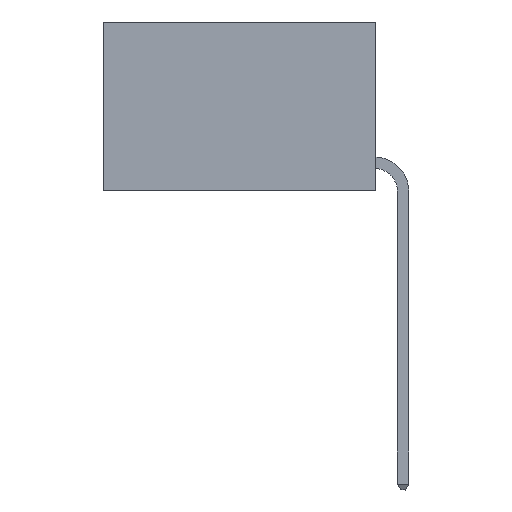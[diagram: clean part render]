
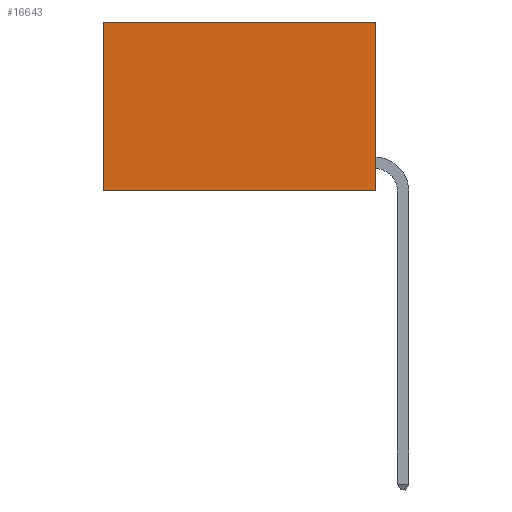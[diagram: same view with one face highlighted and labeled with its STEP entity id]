
A CAD part, left-side view. The second image highlights one B-rep face of the part: STEP entity #16643.
In plain terms, the highlighted planar face has unit normal (-1, 0, 0).
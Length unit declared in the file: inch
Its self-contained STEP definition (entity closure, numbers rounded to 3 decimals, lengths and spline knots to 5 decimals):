
#295 = DIRECTION ( 'NONE',  ( 0., 0., -1. ) ) ;
#575 = VECTOR ( 'NONE', #19983, 39.37008 ) ;
#741 = CARTESIAN_POINT ( 'NONE',  ( 0.2625, 0.6, 0. ) ) ;
#855 = VERTEX_POINT ( 'NONE', #15680 ) ;
#1957 = CARTESIAN_POINT ( 'NONE',  ( 0.2625, 0., 0. ) ) ;
#2111 = EDGE_CURVE ( 'NONE', #17604, #12162, #2617, .T. ) ;
#2617 = LINE ( 'NONE', #741, #11077 ) ;
#3905 = VECTOR ( 'NONE', #17880, 39.37008 ) ;
#4151 = EDGE_CURVE ( 'NONE', #9813, #855, #12773, .T. ) ;
#4707 = CARTESIAN_POINT ( 'NONE',  ( 0.2625, 0., 0. ) ) ;
#5472 = PLANE ( 'NONE',  #5773 ) ;
#5773 = AXIS2_PLACEMENT_3D ( 'NONE', #20198, #10527, #295 ) ;
#5957 = VECTOR ( 'NONE', #14330, 39.37008 ) ;
#5994 = DIRECTION ( 'NONE',  ( 0., 0., -1. ) ) ;
#7853 = CARTESIAN_POINT ( 'NONE',  ( 0.2625, 0.6, -0.37 ) ) ;
#7893 = CARTESIAN_POINT ( 'NONE',  ( 0.2625, 0.6, 0. ) ) ;
#8327 = EDGE_LOOP ( 'NONE', ( #21226, #11391, #18848, #16035 ) ) ;
#8675 = CARTESIAN_POINT ( 'NONE',  ( 0.2625, 0., -0.37 ) ) ;
#9660 = FACE_OUTER_BOUND ( 'NONE', #8327, .T. ) ;
#9813 = VERTEX_POINT ( 'NONE', #1957 ) ;
#10527 = DIRECTION ( 'NONE',  ( 1., 0., 0. ) ) ;
#11077 = VECTOR ( 'NONE', #5994, 39.37008 ) ;
#11391 = ORIENTED_EDGE ( 'NONE', *, *, #15274, .F. ) ;
#12162 = VERTEX_POINT ( 'NONE', #7853 ) ;
#12773 = LINE ( 'NONE', #4707, #3905 ) ;
#14330 = DIRECTION ( 'NONE',  ( 0., 1., 0. ) ) ;
#15274 = EDGE_CURVE ( 'NONE', #855, #12162, #17804, .T. ) ;
#15680 = CARTESIAN_POINT ( 'NONE',  ( 0.2625, 0., -0.37 ) ) ;
#16035 = ORIENTED_EDGE ( 'NONE', *, *, #16879, .T. ) ;
#16643 = ADVANCED_FACE ( 'NONE', ( #9660 ), #5472, .F. ) ;
#16879 = EDGE_CURVE ( 'NONE', #9813, #17604, #19510, .T. ) ;
#17604 = VERTEX_POINT ( 'NONE', #7893 ) ;
#17804 = LINE ( 'NONE', #8675, #575 ) ;
#17880 = DIRECTION ( 'NONE',  ( 0., 0., -1. ) ) ;
#18848 = ORIENTED_EDGE ( 'NONE', *, *, #4151, .F. ) ;
#19142 = CARTESIAN_POINT ( 'NONE',  ( 0.2625, 0., 0. ) ) ;
#19510 = LINE ( 'NONE', #19142, #5957 ) ;
#19983 = DIRECTION ( 'NONE',  ( 0., 1., 0. ) ) ;
#20198 = CARTESIAN_POINT ( 'NONE',  ( 0.2625, 0., 0. ) ) ;
#21226 = ORIENTED_EDGE ( 'NONE', *, *, #2111, .T. ) ;
